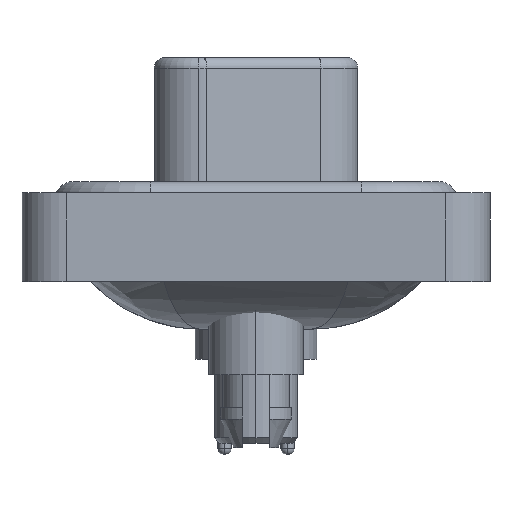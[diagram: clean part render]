
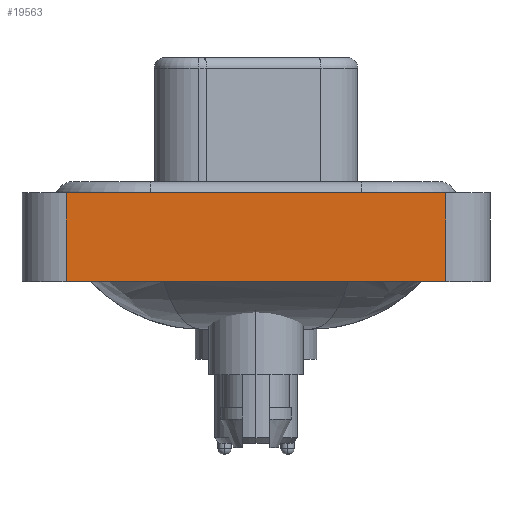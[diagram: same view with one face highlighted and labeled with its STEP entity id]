
A CAD part, left-side view. The second image highlights one B-rep face of the part: STEP entity #19563.
In plain terms, the highlighted planar face has unit normal (-1, 0, 0).
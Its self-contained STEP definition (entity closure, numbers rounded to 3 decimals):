
#164 = DIRECTION ( 'NONE',  ( 0., -1., 0. ) ) ;
#219 = CARTESIAN_POINT ( 'NONE',  ( -7.35, -8.55, -3.6 ) ) ;
#553 = LINE ( 'NONE', #219, #5867 ) ;
#2116 = DIRECTION ( 'NONE',  ( 0., -1., 0. ) ) ;
#3738 = ORIENTED_EDGE ( 'NONE', *, *, #21803, .F. ) ;
#5867 = VECTOR ( 'NONE', #9669, 1000. ) ;
#6155 = DIRECTION ( 'NONE',  ( 0., 0., 1. ) ) ;
#6393 = PLANE ( 'NONE',  #8220 ) ;
#6735 = DIRECTION ( 'NONE',  ( 0., 0., 1. ) ) ;
#6873 = CARTESIAN_POINT ( 'NONE',  ( -7.35, 8.55, 0.4 ) ) ;
#7939 = LINE ( 'NONE', #20596, #16181 ) ;
#8220 = AXIS2_PLACEMENT_3D ( 'NONE', #12076, #15564, #6155 ) ;
#9400 = CARTESIAN_POINT ( 'NONE',  ( -7.35, -8.55, -3.6 ) ) ;
#9669 = DIRECTION ( 'NONE',  ( 0., 0., 1. ) ) ;
#10158 = EDGE_CURVE ( 'NONE', #23229, #23258, #7939, .T. ) ;
#10204 = VERTEX_POINT ( 'NONE', #9400 ) ;
#11442 = EDGE_LOOP ( 'NONE', ( #16700, #17208, #3738, #14979 ) ) ;
#12076 = CARTESIAN_POINT ( 'NONE',  ( -7.35, -8.55, -3.6 ) ) ;
#12079 = EDGE_CURVE ( 'NONE', #12795, #10204, #14949, .T. ) ;
#12795 = VERTEX_POINT ( 'NONE', #14752 ) ;
#13003 = LINE ( 'NONE', #15917, #19034 ) ;
#14752 = CARTESIAN_POINT ( 'NONE',  ( -7.35, 8.55, -3.6 ) ) ;
#14949 = LINE ( 'NONE', #16729, #17276 ) ;
#14979 = ORIENTED_EDGE ( 'NONE', *, *, #12079, .T. ) ;
#15564 = DIRECTION ( 'NONE',  ( -1., 0., 0. ) ) ;
#15917 = CARTESIAN_POINT ( 'NONE',  ( -7.35, 8.55, -3.6 ) ) ;
#16181 = VECTOR ( 'NONE', #2116, 1000. ) ;
#16700 = ORIENTED_EDGE ( 'NONE', *, *, #22887, .T. ) ;
#16729 = CARTESIAN_POINT ( 'NONE',  ( -7.35, -8.55, -3.6 ) ) ;
#17208 = ORIENTED_EDGE ( 'NONE', *, *, #10158, .F. ) ;
#17276 = VECTOR ( 'NONE', #164, 1000. ) ;
#17491 = FACE_OUTER_BOUND ( 'NONE', #11442, .T. ) ;
#19034 = VECTOR ( 'NONE', #6735, 1000. ) ;
#19563 = ADVANCED_FACE ( 'NONE', ( #17491 ), #6393, .T. ) ;
#20596 = CARTESIAN_POINT ( 'NONE',  ( -7.35, -8.55, 0.4 ) ) ;
#21584 = CARTESIAN_POINT ( 'NONE',  ( -7.35, -8.55, 0.4 ) ) ;
#21803 = EDGE_CURVE ( 'NONE', #12795, #23229, #13003, .T. ) ;
#22887 = EDGE_CURVE ( 'NONE', #10204, #23258, #553, .T. ) ;
#23229 = VERTEX_POINT ( 'NONE', #6873 ) ;
#23258 = VERTEX_POINT ( 'NONE', #21584 ) ;
